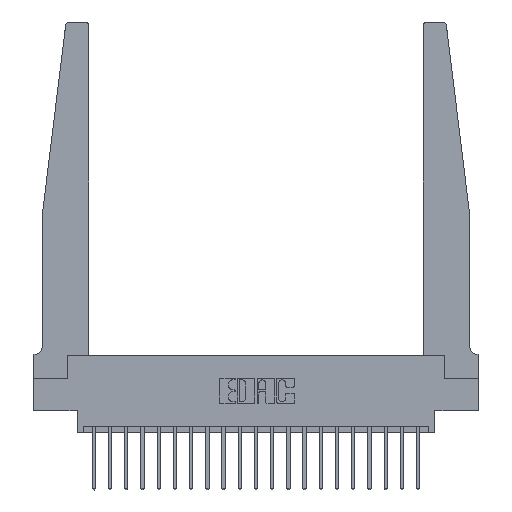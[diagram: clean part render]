
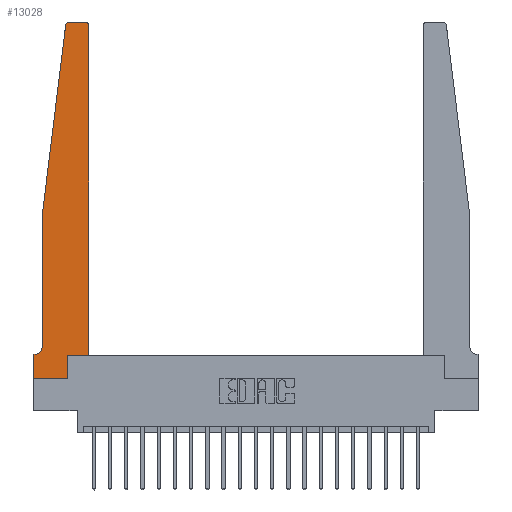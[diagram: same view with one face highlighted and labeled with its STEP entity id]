
A CAD part, top view. The second image highlights one B-rep face of the part: STEP entity #13028.
In plain terms, the highlighted planar face has unit normal (0, 0, 1).
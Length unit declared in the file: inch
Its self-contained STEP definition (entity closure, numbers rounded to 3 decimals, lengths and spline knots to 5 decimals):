
#375 = VERTEX_POINT ( 'NONE', #13261 ) ;
#565 = VERTEX_POINT ( 'NONE', #3802 ) ;
#980 = DIRECTION ( 'NONE',  ( 0., 0., 1. ) ) ;
#1114 = CIRCLE ( 'NONE', #12682, 0.05 ) ;
#1227 = EDGE_CURVE ( 'NONE', #7153, #8651, #5283, .T. ) ;
#1436 = VERTEX_POINT ( 'NONE', #11105 ) ;
#1565 = EDGE_CURVE ( 'NONE', #2368, #10849, #12783, .T. ) ;
#1667 = EDGE_CURVE ( 'NONE', #565, #2368, #19557, .T. ) ;
#2368 = VERTEX_POINT ( 'NONE', #10617 ) ;
#2643 = LINE ( 'NONE', #3831, #15409 ) ;
#2707 = VERTEX_POINT ( 'NONE', #13162 ) ;
#3475 = VERTEX_POINT ( 'NONE', #16797 ) ;
#3802 = CARTESIAN_POINT ( 'NONE',  ( 0.2605, 0., 0.37 ) ) ;
#3831 = CARTESIAN_POINT ( 'NONE',  ( 0.425, 0.18, 0.37 ) ) ;
#3941 = VECTOR ( 'NONE', #6393, 39.37008 ) ;
#4019 = CARTESIAN_POINT ( 'NONE',  ( 0.065, 1.25, 0.37 ) ) ;
#4166 = AXIS2_PLACEMENT_3D ( 'NONE', #9134, #980, #12575 ) ;
#4229 = CARTESIAN_POINT ( 'NONE',  ( 0., 0., 0.37 ) ) ;
#4308 = CARTESIAN_POINT ( 'NONE',  ( 0.015, 0.2375, 0.37 ) ) ;
#4503 = ORIENTED_EDGE ( 'NONE', *, *, #16453, .T. ) ;
#4821 = DIRECTION ( 'NONE',  ( 0., 0., 1. ) ) ;
#4843 = DIRECTION ( 'NONE',  ( -1., 0., 0. ) ) ;
#5162 = LINE ( 'NONE', #18144, #9006 ) ;
#5283 = LINE ( 'NONE', #18839, #18006 ) ;
#5515 = VECTOR ( 'NONE', #20795, 39.37008 ) ;
#5518 = DIRECTION ( 'NONE',  ( 0., 1., 0. ) ) ;
#5526 = DIRECTION ( 'NONE',  ( -0.122, -0.992, 0. ) ) ;
#5937 = LINE ( 'NONE', #8828, #9803 ) ;
#5976 = DIRECTION ( 'NONE',  ( -1., 0., 0. ) ) ;
#6108 = LINE ( 'NONE', #8173, #9462 ) ;
#6393 = DIRECTION ( 'NONE',  ( 1., 0., 0. ) ) ;
#6673 = DIRECTION ( 'NONE',  ( 0., 1., 0. ) ) ;
#7153 = VERTEX_POINT ( 'NONE', #20740 ) ;
#7954 = CARTESIAN_POINT ( 'NONE',  ( 0.395, 2.72, 0.37 ) ) ;
#8173 = CARTESIAN_POINT ( 'NONE',  ( 0.065, 0.1875, 0.37 ) ) ;
#8521 = CARTESIAN_POINT ( 'NONE',  ( 0.27653, 2.75, 0.37 ) ) ;
#8651 = VERTEX_POINT ( 'NONE', #12586 ) ;
#8797 = CIRCLE ( 'NONE', #11844, 0.03 ) ;
#8828 = CARTESIAN_POINT ( 'NONE',  ( 0.065, 1.25, 0.37 ) ) ;
#8871 = ORIENTED_EDGE ( 'NONE', *, *, #1667, .T. ) ;
#9006 = VECTOR ( 'NONE', #4843, 39.37008 ) ;
#9064 = VERTEX_POINT ( 'NONE', #13978 ) ;
#9134 = CARTESIAN_POINT ( 'NONE',  ( 0., 0.1875, 0.37 ) ) ;
#9462 = VECTOR ( 'NONE', #18148, 39.37008 ) ;
#9612 = DIRECTION ( 'NONE',  ( 1., 0., 0. ) ) ;
#9803 = VECTOR ( 'NONE', #5526, 39.37008 ) ;
#9969 = ORIENTED_EDGE ( 'NONE', *, *, #1565, .T. ) ;
#10154 = VECTOR ( 'NONE', #6673, 39.37008 ) ;
#10607 = DIRECTION ( 'NONE',  ( 0., -1., 0. ) ) ;
#10617 = CARTESIAN_POINT ( 'NONE',  ( 0.2605, 0.18, 0.37 ) ) ;
#10849 = VERTEX_POINT ( 'NONE', #18975 ) ;
#10892 = PLANE ( 'NONE',  #4166 ) ;
#11105 = CARTESIAN_POINT ( 'NONE',  ( 0.395, 2.75, 0.37 ) ) ;
#11844 = AXIS2_PLACEMENT_3D ( 'NONE', #14797, #4821, #16458 ) ;
#12054 = EDGE_CURVE ( 'NONE', #1436, #19867, #5162, .T. ) ;
#12303 = VECTOR ( 'NONE', #10607, 39.37008 ) ;
#12575 = DIRECTION ( 'NONE',  ( 1., 0., 0. ) ) ;
#12586 = CARTESIAN_POINT ( 'NONE',  ( 0., 0., 0.37 ) ) ;
#12615 = CIRCLE ( 'NONE', #21218, 0.03 ) ;
#12682 = AXIS2_PLACEMENT_3D ( 'NONE', #4308, #15944, #5976 ) ;
#12783 = LINE ( 'NONE', #16357, #3941 ) ;
#12960 = VERTEX_POINT ( 'NONE', #20575 ) ;
#13028 = ADVANCED_FACE ( 'NONE', ( #15013 ), #10892, .T. ) ;
#13107 = ORIENTED_EDGE ( 'NONE', *, *, #17553, .T. ) ;
#13162 = CARTESIAN_POINT ( 'NONE',  ( 0.24675, 2.72367, 0.37 ) ) ;
#13261 = CARTESIAN_POINT ( 'NONE',  ( 0.425, 2.72, 0.37 ) ) ;
#13282 = CARTESIAN_POINT ( 'NONE',  ( 0.2605, 0.18, 0.37 ) ) ;
#13840 = LINE ( 'NONE', #4229, #5515 ) ;
#13968 = EDGE_CURVE ( 'NONE', #9064, #7153, #6108, .T. ) ;
#13978 = CARTESIAN_POINT ( 'NONE',  ( 0.015, 0.1875, 0.37 ) ) ;
#14407 = ORIENTED_EDGE ( 'NONE', *, *, #12054, .T. ) ;
#14532 = EDGE_CURVE ( 'NONE', #12960, #3475, #21153, .T. ) ;
#14797 = CARTESIAN_POINT ( 'NONE',  ( 0.27653, 2.72, 0.37 ) ) ;
#15013 = FACE_OUTER_BOUND ( 'NONE', #16069, .T. ) ;
#15215 = ORIENTED_EDGE ( 'NONE', *, *, #20923, .T. ) ;
#15409 = VECTOR ( 'NONE', #5518, 39.37008 ) ;
#15712 = ORIENTED_EDGE ( 'NONE', *, *, #18577, .T. ) ;
#15944 = DIRECTION ( 'NONE',  ( 0., 0., -1. ) ) ;
#16069 = EDGE_LOOP ( 'NONE', ( #14407, #15712, #16233, #17510, #18312, #20395, #21402, #4503, #8871, #9969, #13107, #15215 ) ) ;
#16233 = ORIENTED_EDGE ( 'NONE', *, *, #19424, .T. ) ;
#16357 = CARTESIAN_POINT ( 'NONE',  ( 0.425, 0.18, 0.37 ) ) ;
#16453 = EDGE_CURVE ( 'NONE', #8651, #565, #13840, .T. ) ;
#16458 = DIRECTION ( 'NONE',  ( 1., 0., 0. ) ) ;
#16481 = EDGE_CURVE ( 'NONE', #3475, #9064, #1114, .T. ) ;
#16797 = CARTESIAN_POINT ( 'NONE',  ( 0.065, 0.2375, 0.37 ) ) ;
#17510 = ORIENTED_EDGE ( 'NONE', *, *, #14532, .T. ) ;
#17553 = EDGE_CURVE ( 'NONE', #10849, #375, #2643, .T. ) ;
#18006 = VECTOR ( 'NONE', #20498, 39.37008 ) ;
#18144 = CARTESIAN_POINT ( 'NONE',  ( 0.25, 2.75, 0.37 ) ) ;
#18148 = DIRECTION ( 'NONE',  ( -1., 0., 0. ) ) ;
#18312 = ORIENTED_EDGE ( 'NONE', *, *, #16481, .T. ) ;
#18577 = EDGE_CURVE ( 'NONE', #19867, #2707, #8797, .T. ) ;
#18839 = CARTESIAN_POINT ( 'NONE',  ( 0., 0., 0.37 ) ) ;
#18975 = CARTESIAN_POINT ( 'NONE',  ( 0.425, 0.18, 0.37 ) ) ;
#19424 = EDGE_CURVE ( 'NONE', #2707, #12960, #5937, .T. ) ;
#19557 = LINE ( 'NONE', #13282, #10154 ) ;
#19601 = DIRECTION ( 'NONE',  ( 0., 0., 1. ) ) ;
#19867 = VERTEX_POINT ( 'NONE', #8521 ) ;
#20395 = ORIENTED_EDGE ( 'NONE', *, *, #13968, .T. ) ;
#20498 = DIRECTION ( 'NONE',  ( 0., -1., 0. ) ) ;
#20575 = CARTESIAN_POINT ( 'NONE',  ( 0.065, 1.25, 0.37 ) ) ;
#20740 = CARTESIAN_POINT ( 'NONE',  ( 0., 0.1875, 0.37 ) ) ;
#20795 = DIRECTION ( 'NONE',  ( 1., 0., 0. ) ) ;
#20923 = EDGE_CURVE ( 'NONE', #375, #1436, #12615, .T. ) ;
#21153 = LINE ( 'NONE', #4019, #12303 ) ;
#21218 = AXIS2_PLACEMENT_3D ( 'NONE', #7954, #19601, #9612 ) ;
#21402 = ORIENTED_EDGE ( 'NONE', *, *, #1227, .T. ) ;
